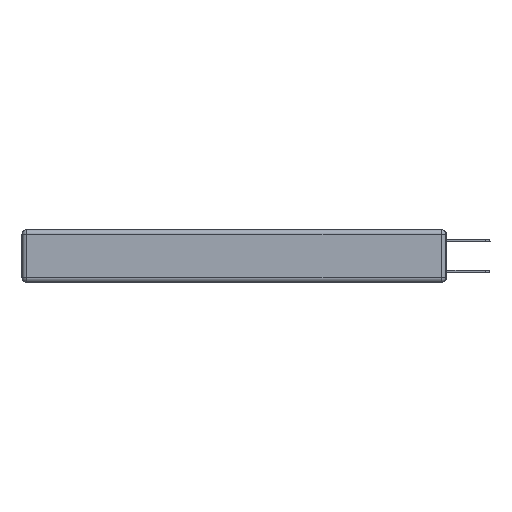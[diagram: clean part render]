
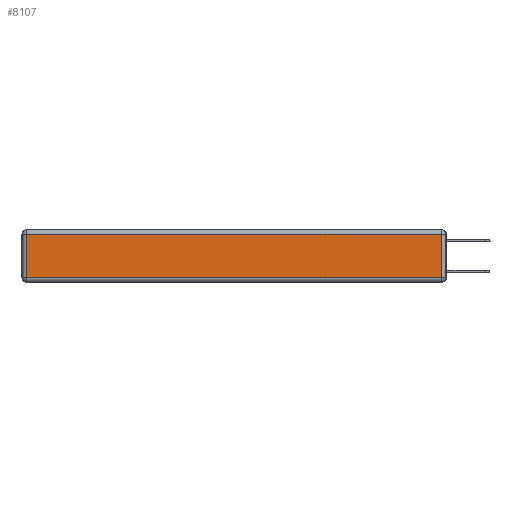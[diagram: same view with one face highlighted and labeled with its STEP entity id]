
A CAD part, left-side view. The second image highlights one B-rep face of the part: STEP entity #8107.
In plain terms, the highlighted planar face has unit normal (-1, 0, 0).
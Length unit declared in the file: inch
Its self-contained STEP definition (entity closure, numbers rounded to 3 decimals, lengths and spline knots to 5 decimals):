
#60 = CARTESIAN_POINT ( 'NONE',  ( 0., 0., -0.313 ) ) ;
#153 = CARTESIAN_POINT ( 'NONE',  ( 0., 0.03, -0.313 ) ) ;
#912 = LINE ( 'NONE', #8808, #1922 ) ;
#1044 = PLANE ( 'NONE',  #24637 ) ;
#1062 = ORIENTED_EDGE ( 'NONE', *, *, #8038, .T. ) ;
#1922 = VECTOR ( 'NONE', #14743, 39.37008 ) ;
#3283 = VECTOR ( 'NONE', #18010, 39.37008 ) ;
#4133 = VERTEX_POINT ( 'NONE', #24790 ) ;
#4395 = ORIENTED_EDGE ( 'NONE', *, *, #21165, .T. ) ;
#4652 = CARTESIAN_POINT ( 'NONE',  ( 0., 2.72, -0.343 ) ) ;
#5515 = EDGE_CURVE ( 'NONE', #20423, #13738, #17764, .T. ) ;
#8038 = EDGE_CURVE ( 'NONE', #4133, #14911, #912, .T. ) ;
#8107 = ADVANCED_FACE ( 'NONE', ( #10885 ), #1044, .T. ) ;
#8132 = LINE ( 'NONE', #4652, #9085 ) ;
#8719 = ORIENTED_EDGE ( 'NONE', *, *, #8866, .T. ) ;
#8808 = CARTESIAN_POINT ( 'NONE',  ( 0., 2.75, -0.03 ) ) ;
#8866 = EDGE_CURVE ( 'NONE', #13738, #4133, #14804, .T. ) ;
#9085 = VECTOR ( 'NONE', #20256, 39.37008 ) ;
#10885 = FACE_OUTER_BOUND ( 'NONE', #19965, .T. ) ;
#10950 = CARTESIAN_POINT ( 'NONE',  ( 0., 0.03, -0.343 ) ) ;
#13215 = VECTOR ( 'NONE', #22690, 39.37008 ) ;
#13738 = VERTEX_POINT ( 'NONE', #153 ) ;
#14743 = DIRECTION ( 'NONE',  ( 0., 1., 0. ) ) ;
#14804 = LINE ( 'NONE', #10950, #13215 ) ;
#14871 = DIRECTION ( 'NONE',  ( -1., 0., 0. ) ) ;
#14911 = VERTEX_POINT ( 'NONE', #25396 ) ;
#15109 = CARTESIAN_POINT ( 'NONE',  ( 0., 0., -0.343 ) ) ;
#15137 = CARTESIAN_POINT ( 'NONE',  ( 0., 2.72, -0.313 ) ) ;
#17764 = LINE ( 'NONE', #60, #3283 ) ;
#18010 = DIRECTION ( 'NONE',  ( 0., -1., 0. ) ) ;
#19965 = EDGE_LOOP ( 'NONE', ( #24629, #8719, #1062, #4395 ) ) ;
#20256 = DIRECTION ( 'NONE',  ( 0., 0., -1. ) ) ;
#20423 = VERTEX_POINT ( 'NONE', #15137 ) ;
#21165 = EDGE_CURVE ( 'NONE', #14911, #20423, #8132, .T. ) ;
#22690 = DIRECTION ( 'NONE',  ( 0., 0., 1. ) ) ;
#22875 = DIRECTION ( 'NONE',  ( 0., 0., 1. ) ) ;
#24629 = ORIENTED_EDGE ( 'NONE', *, *, #5515, .T. ) ;
#24637 = AXIS2_PLACEMENT_3D ( 'NONE', #15109, #14871, #22875 ) ;
#24790 = CARTESIAN_POINT ( 'NONE',  ( 0., 0.03, -0.03 ) ) ;
#25396 = CARTESIAN_POINT ( 'NONE',  ( 0., 2.72, -0.03 ) ) ;
